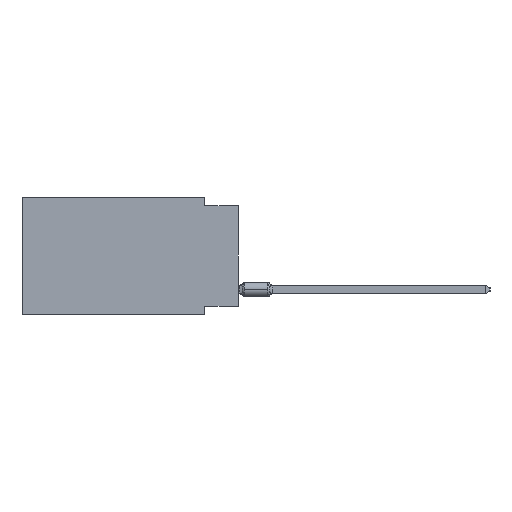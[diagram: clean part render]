
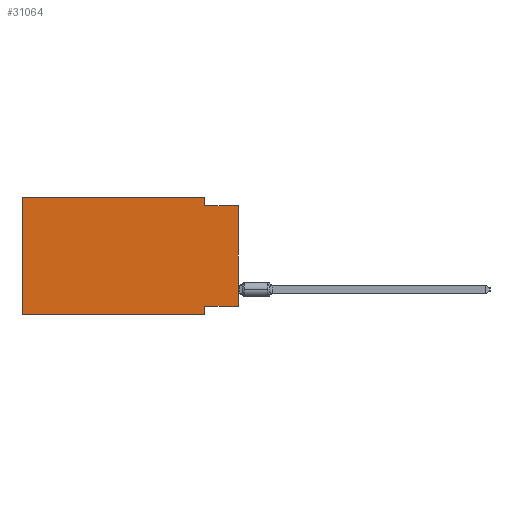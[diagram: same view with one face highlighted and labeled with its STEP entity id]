
A CAD part, left-side view. The second image highlights one B-rep face of the part: STEP entity #31064.
In plain terms, the highlighted planar face has unit normal (-1, 0, 0).
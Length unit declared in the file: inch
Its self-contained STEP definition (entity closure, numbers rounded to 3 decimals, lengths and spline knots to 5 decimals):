
#474 = EDGE_CURVE ( 'NONE', #13257, #56035, #16012, .T. ) ;
#1744 = PLANE ( 'NONE',  #53514 ) ;
#2995 = VERTEX_POINT ( 'NONE', #52984 ) ;
#3821 = ORIENTED_EDGE ( 'NONE', *, *, #36037, .F. ) ;
#5055 = VERTEX_POINT ( 'NONE', #7332 ) ;
#5165 = VERTEX_POINT ( 'NONE', #30022 ) ;
#7332 = CARTESIAN_POINT ( 'NONE',  ( 0., 0.645, 0. ) ) ;
#8118 = DIRECTION ( 'NONE',  ( 0., -1., 0. ) ) ;
#8254 = DIRECTION ( 'NONE',  ( 0., 0., -1. ) ) ;
#8729 = VERTEX_POINT ( 'NONE', #30919 ) ;
#9280 = CARTESIAN_POINT ( 'NONE',  ( 0., 0.645, 0. ) ) ;
#9534 = VECTOR ( 'NONE', #46717, 39.37008 ) ;
#9880 = EDGE_LOOP ( 'NONE', ( #14972, #37778, #54889, #20111, #35994, #55396, #32553, #3821 ) ) ;
#13257 = VERTEX_POINT ( 'NONE', #15827 ) ;
#14170 = CARTESIAN_POINT ( 'NONE',  ( 0., 0., -0.325 ) ) ;
#14356 = LINE ( 'NONE', #14630, #33050 ) ;
#14630 = CARTESIAN_POINT ( 'NONE',  ( 0., 0.1, 0. ) ) ;
#14777 = EDGE_CURVE ( 'NONE', #25473, #5055, #39732, .T. ) ;
#14972 = ORIENTED_EDGE ( 'NONE', *, *, #41388, .T. ) ;
#15827 = CARTESIAN_POINT ( 'NONE',  ( 0., 0.1, -0.025 ) ) ;
#16012 = LINE ( 'NONE', #46739, #29455 ) ;
#16269 = LINE ( 'NONE', #33243, #22076 ) ;
#18921 = LINE ( 'NONE', #40766, #53062 ) ;
#19234 = DIRECTION ( 'NONE',  ( 0., 0., -1. ) ) ;
#20111 = ORIENTED_EDGE ( 'NONE', *, *, #38376, .F. ) ;
#22076 = VECTOR ( 'NONE', #51320, 39.37008 ) ;
#25473 = VERTEX_POINT ( 'NONE', #45968 ) ;
#25486 = LINE ( 'NONE', #30087, #51292 ) ;
#29455 = VECTOR ( 'NONE', #29814, 39.37008 ) ;
#29814 = DIRECTION ( 'NONE',  ( 0., -1., 0. ) ) ;
#30022 = CARTESIAN_POINT ( 'NONE',  ( 0., 0.1, -0.325 ) ) ;
#30087 = CARTESIAN_POINT ( 'NONE',  ( 0., 0.1, -0.35 ) ) ;
#30215 = CARTESIAN_POINT ( 'NONE',  ( 0., 0.645, -0.35 ) ) ;
#30919 = CARTESIAN_POINT ( 'NONE',  ( 0., 0.1, 0. ) ) ;
#31064 = ADVANCED_FACE ( 'NONE', ( #41092 ), #1744, .F. ) ;
#32553 = ORIENTED_EDGE ( 'NONE', *, *, #53604, .F. ) ;
#33050 = VECTOR ( 'NONE', #45085, 39.37008 ) ;
#33243 = CARTESIAN_POINT ( 'NONE',  ( 0., 0., 0. ) ) ;
#34342 = LINE ( 'NONE', #14170, #56698 ) ;
#35259 = EDGE_CURVE ( 'NONE', #25473, #2995, #47460, .T. ) ;
#35946 = CARTESIAN_POINT ( 'NONE',  ( 0., 0., -0.025 ) ) ;
#35994 = ORIENTED_EDGE ( 'NONE', *, *, #14777, .F. ) ;
#36037 = EDGE_CURVE ( 'NONE', #56570, #5165, #34342, .T. ) ;
#37331 = VECTOR ( 'NONE', #8118, 39.37008 ) ;
#37778 = ORIENTED_EDGE ( 'NONE', *, *, #474, .F. ) ;
#38376 = EDGE_CURVE ( 'NONE', #5055, #8729, #18921, .T. ) ;
#39732 = LINE ( 'NONE', #9280, #9534 ) ;
#39756 = DIRECTION ( 'NONE',  ( 0., 1., 0. ) ) ;
#40737 = EDGE_CURVE ( 'NONE', #8729, #13257, #14356, .T. ) ;
#40766 = CARTESIAN_POINT ( 'NONE',  ( 0., 0.645, 0. ) ) ;
#40800 = CARTESIAN_POINT ( 'NONE',  ( 0., 0.645, 0. ) ) ;
#41092 = FACE_OUTER_BOUND ( 'NONE', #9880, .T. ) ;
#41388 = EDGE_CURVE ( 'NONE', #56570, #56035, #16269, .T. ) ;
#45085 = DIRECTION ( 'NONE',  ( 0., 0., -1. ) ) ;
#45948 = DIRECTION ( 'NONE',  ( 1., 0., 0. ) ) ;
#45968 = CARTESIAN_POINT ( 'NONE',  ( 0., 0.645, -0.35 ) ) ;
#46717 = DIRECTION ( 'NONE',  ( 0., 0., 1. ) ) ;
#46739 = CARTESIAN_POINT ( 'NONE',  ( 0., 0., -0.025 ) ) ;
#47460 = LINE ( 'NONE', #30215, #37331 ) ;
#49104 = DIRECTION ( 'NONE',  ( 0., -1., 0. ) ) ;
#50201 = CARTESIAN_POINT ( 'NONE',  ( 0., 0., -0.325 ) ) ;
#51292 = VECTOR ( 'NONE', #8254, 39.37008 ) ;
#51320 = DIRECTION ( 'NONE',  ( 0., 0., 1. ) ) ;
#52984 = CARTESIAN_POINT ( 'NONE',  ( 0., 0.1, -0.35 ) ) ;
#53062 = VECTOR ( 'NONE', #49104, 39.37008 ) ;
#53514 = AXIS2_PLACEMENT_3D ( 'NONE', #40800, #45948, #19234 ) ;
#53604 = EDGE_CURVE ( 'NONE', #5165, #2995, #25486, .T. ) ;
#54889 = ORIENTED_EDGE ( 'NONE', *, *, #40737, .F. ) ;
#55396 = ORIENTED_EDGE ( 'NONE', *, *, #35259, .T. ) ;
#56035 = VERTEX_POINT ( 'NONE', #35946 ) ;
#56570 = VERTEX_POINT ( 'NONE', #50201 ) ;
#56698 = VECTOR ( 'NONE', #39756, 39.37008 ) ;
